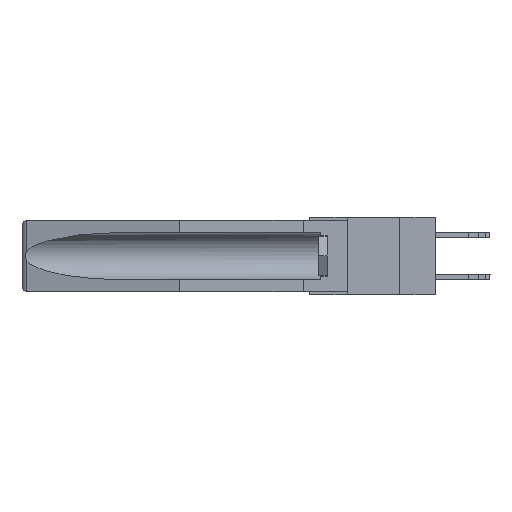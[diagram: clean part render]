
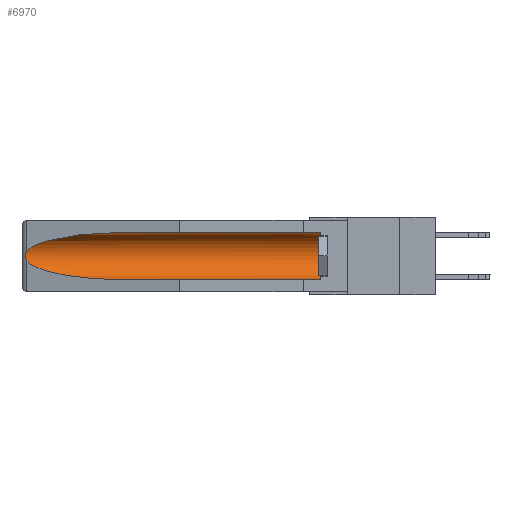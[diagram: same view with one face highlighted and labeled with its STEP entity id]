
A CAD part, left-side view. The second image highlights one B-rep face of the part: STEP entity #6970.
In plain terms, the highlighted cylindrical face has radius 2.857 mm (diameter 5.715 mm), a partial arc.
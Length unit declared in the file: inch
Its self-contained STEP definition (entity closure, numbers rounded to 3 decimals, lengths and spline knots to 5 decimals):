
#407 = CARTESIAN_POINT ( 'NONE',  ( 0.155, -0.30754, -0.1715 ) ) ;
#659 = AXIS2_PLACEMENT_3D ( 'NONE', #407, #10650, #10833 ) ;
#832 = ORIENTED_EDGE ( 'NONE', *, *, #8577, .T. ) ;
#1193 = CARTESIAN_POINT ( 'NONE',  ( 0.2675, 1.53308, -0.17534 ) ) ;
#1317 =( BOUNDED_CURVE ( )  B_SPLINE_CURVE ( 3, ( #14341, #7165, #8876, #5544 ),
 .UNSPECIFIED., .F., .F. ) 
 B_SPLINE_CURVE_WITH_KNOTS ( ( 4, 4 ),
 ( 4.71239, 6.08839 ),
 .UNSPECIFIED. ) 
 CURVE ( )  GEOMETRIC_REPRESENTATION_ITEM ( )  RATIONAL_B_SPLINE_CURVE ( ( 1., 0.848, 0.848, 1. ) ) 
 REPRESENTATION_ITEM ( '' )  );
#1708 = DIRECTION ( 'NONE',  ( 0., -1., 0. ) ) ;
#1762 = ORIENTED_EDGE ( 'NONE', *, *, #12643, .F. ) ;
#1957 = ORIENTED_EDGE ( 'NONE', *, *, #10227, .T. ) ;
#2129 = CARTESIAN_POINT ( 'NONE',  ( 0.155, 0.126, -0.284 ) ) ;
#2302 = CARTESIAN_POINT ( 'NONE',  ( 0.155, -0.30754, -0.059 ) ) ;
#2627 = LINE ( 'NONE', #2302, #18690 ) ;
#2652 = CARTESIAN_POINT ( 'NONE',  ( 0.26597, 1.5296, -0.19026 ) ) ;
#3106 = EDGE_CURVE ( 'NONE', #12354, #18075, #1317, .T. ) ;
#3174 = ORIENTED_EDGE ( 'NONE', *, *, #12438, .T. ) ;
#3235 = CARTESIAN_POINT ( 'NONE',  ( 0.155, 1.07973, -0.059 ) ) ;
#3818 = CARTESIAN_POINT ( 'NONE',  ( 0.26597, 1.52961, -0.15275 ) ) ;
#4282 = CARTESIAN_POINT ( 'NONE',  ( 0.155, 1.07973, -0.284 ) ) ;
#4803 = VERTEX_POINT ( 'NONE', #17673 ) ;
#5164 = CARTESIAN_POINT ( 'NONE',  ( 0.26537, 1.52718, -0.19328 ) ) ;
#5403 = CARTESIAN_POINT ( 'NONE',  ( 0.26537, 1.52718, -0.19328 ) ) ;
#5544 = CARTESIAN_POINT ( 'NONE',  ( 0.26537, 1.52718, -0.14972 ) ) ;
#6692 = AXIS2_PLACEMENT_3D ( 'NONE', #11901, #1708, #16258 ) ;
#6970 = ADVANCED_FACE ( 'NONE', ( #18948 ), #12092, .F. ) ;
#7165 = CARTESIAN_POINT ( 'NONE',  ( 0.21114, 1.30732, -0.059 ) ) ;
#7434 = EDGE_CURVE ( 'NONE', #4803, #12354, #2627, .T. ) ;
#7676 = CARTESIAN_POINT ( 'NONE',  ( 0.155, -0.30754, -0.284 ) ) ;
#7743 = VERTEX_POINT ( 'NONE', #2129 ) ;
#8547 = CARTESIAN_POINT ( 'NONE',  ( 0.21114, 1.30732, -0.284 ) ) ;
#8568 = LINE ( 'NONE', #7676, #14021 ) ;
#8577 = EDGE_CURVE ( 'NONE', #18075, #10097, #17789, .T. ) ;
#8876 = CARTESIAN_POINT ( 'NONE',  ( 0.25451, 1.48313, -0.09465 ) ) ;
#9339 = CARTESIAN_POINT ( 'NONE',  ( 0.26537, 1.52718, -0.14972 ) ) ;
#10097 = VERTEX_POINT ( 'NONE', #16062 ) ;
#10227 = EDGE_CURVE ( 'NONE', #7743, #4803, #15984, .T. ) ;
#10650 = DIRECTION ( 'NONE',  ( 0., 1., 0. ) ) ;
#10833 = DIRECTION ( 'NONE',  ( 0., 0., 1. ) ) ;
#10937 = ORIENTED_EDGE ( 'NONE', *, *, #7434, .T. ) ;
#11201 = CARTESIAN_POINT ( 'NONE',  ( 0.2673, 1.5327, -0.16383 ) ) ;
#11451 = CARTESIAN_POINT ( 'NONE',  ( 0.26655, 1.53094, -0.18657 ) ) ;
#11901 = CARTESIAN_POINT ( 'NONE',  ( 0.155, 0.126, -0.1715 ) ) ;
#12089 = DIRECTION ( 'NONE',  ( 0., 1., 0. ) ) ;
#12092 = CYLINDRICAL_SURFACE ( 'NONE', #659, 0.1125 ) ;
#12354 = VERTEX_POINT ( 'NONE', #3235 ) ;
#12438 = EDGE_CURVE ( 'NONE', #10097, #17953, #17537, .T. ) ;
#12478 = DIRECTION ( 'NONE',  ( 0., 1., 0. ) ) ;
#12643 = EDGE_CURVE ( 'NONE', #7743, #17953, #8568, .T. ) ;
#13247 = ORIENTED_EDGE ( 'NONE', *, *, #3106, .T. ) ;
#14021 = VECTOR ( 'NONE', #12089, 39.37008 ) ;
#14313 = CARTESIAN_POINT ( 'NONE',  ( 0.26654, 1.53092, -0.15636 ) ) ;
#14341 = CARTESIAN_POINT ( 'NONE',  ( 0.155, 1.07973, -0.059 ) ) ;
#15039 = CARTESIAN_POINT ( 'NONE',  ( 0.155, 1.07973, -0.284 ) ) ;
#15428 = CARTESIAN_POINT ( 'NONE',  ( 0.25451, 1.48313, -0.24835 ) ) ;
#15984 = CIRCLE ( 'NONE', #6692, 0.1125 ) ;
#16062 = CARTESIAN_POINT ( 'NONE',  ( 0.26537, 1.52718, -0.19328 ) ) ;
#16258 = DIRECTION ( 'NONE',  ( 0., 0., 1. ) ) ;
#16984 = CARTESIAN_POINT ( 'NONE',  ( 0.26537, 1.52718, -0.14972 ) ) ;
#17095 = CARTESIAN_POINT ( 'NONE',  ( 0.2673, 1.53269, -0.17917 ) ) ;
#17537 =( BOUNDED_CURVE ( )  B_SPLINE_CURVE ( 3, ( #5164, #15428, #8547, #4282 ),
 .UNSPECIFIED., .F., .T. ) 
 B_SPLINE_CURVE_WITH_KNOTS ( ( 4, 4 ),
 ( 0.1948, 1.5708 ),
 .UNSPECIFIED. ) 
 CURVE ( )  GEOMETRIC_REPRESENTATION_ITEM ( )  RATIONAL_B_SPLINE_CURVE ( ( 1., 0.848, 0.848, 1. ) ) 
 REPRESENTATION_ITEM ( '' )  );
#17673 = CARTESIAN_POINT ( 'NONE',  ( 0.155, 0.126, -0.059 ) ) ;
#17789 = B_SPLINE_CURVE_WITH_KNOTS ( 'NONE', 3,
 ( #16984, #3818, #14313, #11201, #18757, #1193, #17095, #11451, #2652, #5403 ),
 .UNSPECIFIED., .F., .F.,
 ( 4, 2, 2, 2, 4 ),
 ( 0., 0.00029, 0.00058, 0.00087, 0.00117 ),
 .UNSPECIFIED. ) ;
#17953 = VERTEX_POINT ( 'NONE', #15039 ) ;
#18069 = EDGE_LOOP ( 'NONE', ( #13247, #832, #3174, #1762, #1957, #10937 ) ) ;
#18075 = VERTEX_POINT ( 'NONE', #9339 ) ;
#18690 = VECTOR ( 'NONE', #12478, 39.37008 ) ;
#18757 = CARTESIAN_POINT ( 'NONE',  ( 0.2675, 1.53308, -0.16763 ) ) ;
#18948 = FACE_OUTER_BOUND ( 'NONE', #18069, .T. ) ;
